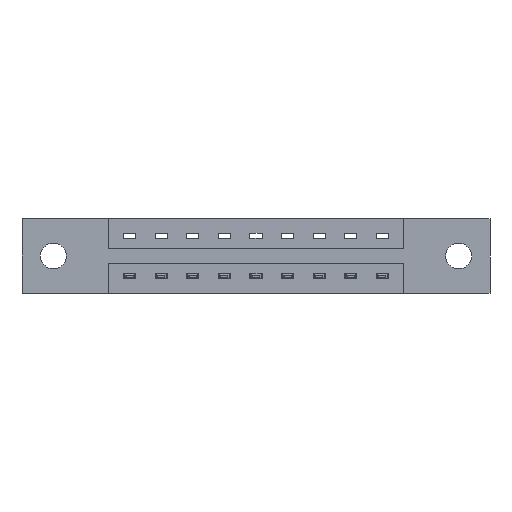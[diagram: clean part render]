
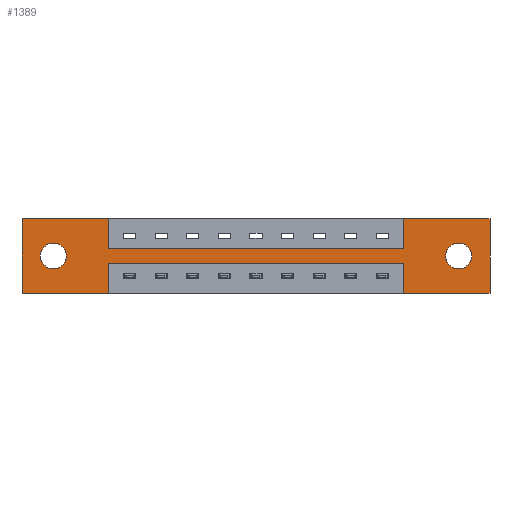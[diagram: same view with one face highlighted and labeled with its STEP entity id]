
A CAD part, front view. The second image highlights one B-rep face of the part: STEP entity #1389.
In plain terms, the highlighted planar face has unit normal (0, -1, 0).
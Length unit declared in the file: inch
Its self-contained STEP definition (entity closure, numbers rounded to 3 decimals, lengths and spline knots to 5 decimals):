
#8 = VECTOR ( 'NONE', #2600, 39.37008 ) ;
#12 = EDGE_CURVE ( 'NONE', #10184, #2739, #1317, .T. ) ;
#14 = EDGE_LOOP ( 'NONE', ( #3819, #10379 ) ) ;
#52 = ORIENTED_EDGE ( 'NONE', *, *, #6218, .T. ) ;
#67 = EDGE_LOOP ( 'NONE', ( #52, #2562 ) ) ;
#458 = VERTEX_POINT ( 'NONE', #7174 ) ;
#569 = EDGE_CURVE ( 'NONE', #7236, #9083, #9987, .T. ) ;
#582 = CARTESIAN_POINT ( 'NONE',  ( 0., 0., 0. ) ) ;
#648 = ORIENTED_EDGE ( 'NONE', *, *, #5419, .F. ) ;
#692 = VECTOR ( 'NONE', #4787, 39.37008 ) ;
#770 = EDGE_CURVE ( 'NONE', #9083, #9207, #10099, .T. ) ;
#872 = VECTOR ( 'NONE', #1946, 39.37008 ) ;
#923 = AXIS2_PLACEMENT_3D ( 'NONE', #2816, #2030, #1575 ) ;
#1024 = CARTESIAN_POINT ( 'NONE',  ( 1.885, 0., 0. ) ) ;
#1047 = CARTESIAN_POINT ( 'NONE',  ( 1.885, 0., -0.15 ) ) ;
#1225 = ORIENTED_EDGE ( 'NONE', *, *, #3499, .F. ) ;
#1302 = CARTESIAN_POINT ( 'NONE',  ( 2.31, 0., 0. ) ) ;
#1317 = LINE ( 'NONE', #1812, #9880 ) ;
#1385 = ORIENTED_EDGE ( 'NONE', *, *, #7901, .F. ) ;
#1389 = ADVANCED_FACE ( 'NONE', ( #9699, #5748, #8130 ), #2143, .T. ) ;
#1575 = DIRECTION ( 'NONE',  ( 0., 0., -1. ) ) ;
#1652 = DIRECTION ( 'NONE',  ( 0., 0., -1. ) ) ;
#1812 = CARTESIAN_POINT ( 'NONE',  ( 1.885, 0., -0.37 ) ) ;
#1946 = DIRECTION ( 'NONE',  ( -1., 0., 0. ) ) ;
#1984 = ORIENTED_EDGE ( 'NONE', *, *, #569, .F. ) ;
#2030 = DIRECTION ( 'NONE',  ( 0., -1., 0. ) ) ;
#2089 = VECTOR ( 'NONE', #8430, 39.37008 ) ;
#2143 = PLANE ( 'NONE',  #923 ) ;
#2194 = VECTOR ( 'NONE', #6625, 39.37008 ) ;
#2396 = CARTESIAN_POINT ( 'NONE',  ( 2.155, 0., -0.185 ) ) ;
#2562 = ORIENTED_EDGE ( 'NONE', *, *, #2701, .T. ) ;
#2600 = DIRECTION ( 'NONE',  ( 0., 0., 1. ) ) ;
#2699 = VERTEX_POINT ( 'NONE', #6415 ) ;
#2701 = EDGE_CURVE ( 'NONE', #4265, #8210, #3915, .T. ) ;
#2739 = VERTEX_POINT ( 'NONE', #5253 ) ;
#2797 = LINE ( 'NONE', #10108, #8 ) ;
#2814 = DIRECTION ( 'NONE',  ( 0., 0., 1. ) ) ;
#2816 = CARTESIAN_POINT ( 'NONE',  ( 0., 0., -0.37 ) ) ;
#2850 = ORIENTED_EDGE ( 'NONE', *, *, #7556, .F. ) ;
#3068 = CARTESIAN_POINT ( 'NONE',  ( 2.155, 0., -0.121 ) ) ;
#3204 = EDGE_CURVE ( 'NONE', #6936, #6884, #4412, .T. ) ;
#3317 = DIRECTION ( 'NONE',  ( 1., 0., 0. ) ) ;
#3389 = DIRECTION ( 'NONE',  ( 1., 0., 0. ) ) ;
#3407 = ORIENTED_EDGE ( 'NONE', *, *, #7855, .F. ) ;
#3423 = EDGE_CURVE ( 'NONE', #2699, #4087, #2797, .T. ) ;
#3446 = DIRECTION ( 'NONE',  ( 0., 0., -1. ) ) ;
#3473 = DIRECTION ( 'NONE',  ( 0., 1., 0. ) ) ;
#3483 = DIRECTION ( 'NONE',  ( 0., 1., 0. ) ) ;
#3499 = EDGE_CURVE ( 'NONE', #7143, #10184, #8337, .T. ) ;
#3549 = DIRECTION ( 'NONE',  ( 0., 0., 1. ) ) ;
#3565 = CIRCLE ( 'NONE', #8037, 0.064 ) ;
#3625 = DIRECTION ( 'NONE',  ( 0., 0., -1. ) ) ;
#3819 = ORIENTED_EDGE ( 'NONE', *, *, #7122, .T. ) ;
#3915 = CIRCLE ( 'NONE', #8149, 0.064 ) ;
#3932 = EDGE_CURVE ( 'NONE', #4850, #9013, #4812, .T. ) ;
#4087 = VERTEX_POINT ( 'NONE', #9113 ) ;
#4117 = CARTESIAN_POINT ( 'NONE',  ( 0.155, 0., -0.121 ) ) ;
#4147 = AXIS2_PLACEMENT_3D ( 'NONE', #2396, #3473, #3446 ) ;
#4148 = CARTESIAN_POINT ( 'NONE',  ( 1.885, 0., -0.37 ) ) ;
#4151 = CARTESIAN_POINT ( 'NONE',  ( 0.155, 0., -0.249 ) ) ;
#4265 = VERTEX_POINT ( 'NONE', #4151 ) ;
#4383 = EDGE_CURVE ( 'NONE', #9013, #7143, #9272, .T. ) ;
#4412 = LINE ( 'NONE', #7427, #2089 ) ;
#4546 = VECTOR ( 'NONE', #6333, 39.37008 ) ;
#4554 = EDGE_CURVE ( 'NONE', #458, #9960, #8317, .T. ) ;
#4787 = DIRECTION ( 'NONE',  ( 1., 0., 0. ) ) ;
#4812 = LINE ( 'NONE', #8941, #5062 ) ;
#4850 = VERTEX_POINT ( 'NONE', #8526 ) ;
#5061 = VECTOR ( 'NONE', #9419, 39.37008 ) ;
#5062 = VECTOR ( 'NONE', #3317, 39.37008 ) ;
#5115 = ORIENTED_EDGE ( 'NONE', *, *, #3204, .F. ) ;
#5125 = ORIENTED_EDGE ( 'NONE', *, *, #3423, .F. ) ;
#5248 = ORIENTED_EDGE ( 'NONE', *, *, #3932, .F. ) ;
#5253 = CARTESIAN_POINT ( 'NONE',  ( 1.885, 0., -0.22 ) ) ;
#5321 = CARTESIAN_POINT ( 'NONE',  ( 0., 0., -0.37 ) ) ;
#5419 = EDGE_CURVE ( 'NONE', #6884, #2699, #9003, .T. ) ;
#5631 = ORIENTED_EDGE ( 'NONE', *, *, #12, .F. ) ;
#5643 = DIRECTION ( 'NONE',  ( 0., 0., 1. ) ) ;
#5748 = FACE_BOUND ( 'NONE', #67, .T. ) ;
#5768 = EDGE_LOOP ( 'NONE', ( #5115, #3407, #5631, #1225, #8258, #5248, #1385, #6011, #1984, #2850, #5125, #648 ) ) ;
#5794 = CARTESIAN_POINT ( 'NONE',  ( 0.425, 0., -0.15 ) ) ;
#5831 = CARTESIAN_POINT ( 'NONE',  ( 0.155, 0., -0.185 ) ) ;
#6011 = ORIENTED_EDGE ( 'NONE', *, *, #770, .F. ) ;
#6160 = CARTESIAN_POINT ( 'NONE',  ( 0., 0., -0.37 ) ) ;
#6218 = EDGE_CURVE ( 'NONE', #8210, #4265, #3565, .T. ) ;
#6225 = CARTESIAN_POINT ( 'NONE',  ( 0.425, 0., -0.22 ) ) ;
#6227 = VECTOR ( 'NONE', #3389, 39.37008 ) ;
#6239 = CIRCLE ( 'NONE', #4147, 0.064 ) ;
#6274 = DIRECTION ( 'NONE',  ( 0., 1., 0. ) ) ;
#6281 = CARTESIAN_POINT ( 'NONE',  ( 0.155, 0., -0.185 ) ) ;
#6333 = DIRECTION ( 'NONE',  ( -1., 0., 0. ) ) ;
#6415 = CARTESIAN_POINT ( 'NONE',  ( 0., 0., -0.37 ) ) ;
#6625 = DIRECTION ( 'NONE',  ( -1., 0., 0. ) ) ;
#6832 = CARTESIAN_POINT ( 'NONE',  ( 2.31, 0., 0. ) ) ;
#6880 = CARTESIAN_POINT ( 'NONE',  ( 0.425, 0., -0.22 ) ) ;
#6884 = VERTEX_POINT ( 'NONE', #10277 ) ;
#6936 = VERTEX_POINT ( 'NONE', #6880 ) ;
#6989 = CARTESIAN_POINT ( 'NONE',  ( 0.425, 0., 0. ) ) ;
#7091 = DIRECTION ( 'NONE',  ( 0., 1., 0. ) ) ;
#7122 = EDGE_CURVE ( 'NONE', #9960, #458, #6239, .T. ) ;
#7143 = VERTEX_POINT ( 'NONE', #7394 ) ;
#7174 = CARTESIAN_POINT ( 'NONE',  ( 2.155, 0., -0.249 ) ) ;
#7234 = VECTOR ( 'NONE', #7875, 39.37008 ) ;
#7236 = VERTEX_POINT ( 'NONE', #10088 ) ;
#7394 = CARTESIAN_POINT ( 'NONE',  ( 2.31, 0., -0.37 ) ) ;
#7427 = CARTESIAN_POINT ( 'NONE',  ( 0.425, 0., -0.37 ) ) ;
#7556 = EDGE_CURVE ( 'NONE', #4087, #7236, #8336, .T. ) ;
#7744 = CARTESIAN_POINT ( 'NONE',  ( 0.425, 0., -0.15 ) ) ;
#7855 = EDGE_CURVE ( 'NONE', #2739, #6936, #9770, .T. ) ;
#7875 = DIRECTION ( 'NONE',  ( 0., 0., -1. ) ) ;
#7901 = EDGE_CURVE ( 'NONE', #9207, #4850, #9541, .T. ) ;
#8037 = AXIS2_PLACEMENT_3D ( 'NONE', #6281, #6274, #5643 ) ;
#8130 = FACE_OUTER_BOUND ( 'NONE', #5768, .T. ) ;
#8149 = AXIS2_PLACEMENT_3D ( 'NONE', #5831, #3483, #3549 ) ;
#8210 = VERTEX_POINT ( 'NONE', #4117 ) ;
#8258 = ORIENTED_EDGE ( 'NONE', *, *, #4383, .F. ) ;
#8317 = CIRCLE ( 'NONE', #10616, 0.064 ) ;
#8336 = LINE ( 'NONE', #582, #6227 ) ;
#8337 = LINE ( 'NONE', #5321, #4546 ) ;
#8430 = DIRECTION ( 'NONE',  ( 0., 0., -1. ) ) ;
#8441 = VECTOR ( 'NONE', #1652, 39.37008 ) ;
#8526 = CARTESIAN_POINT ( 'NONE',  ( 1.885, 0., 0. ) ) ;
#8582 = CARTESIAN_POINT ( 'NONE',  ( 2.155, 0., -0.185 ) ) ;
#8941 = CARTESIAN_POINT ( 'NONE',  ( 0., 0., 0. ) ) ;
#9003 = LINE ( 'NONE', #6160, #2194 ) ;
#9013 = VERTEX_POINT ( 'NONE', #6832 ) ;
#9083 = VERTEX_POINT ( 'NONE', #7744 ) ;
#9113 = CARTESIAN_POINT ( 'NONE',  ( 0., 0., 0. ) ) ;
#9207 = VERTEX_POINT ( 'NONE', #1047 ) ;
#9272 = LINE ( 'NONE', #1302, #7234 ) ;
#9419 = DIRECTION ( 'NONE',  ( 0., 0., 1. ) ) ;
#9541 = LINE ( 'NONE', #1024, #5061 ) ;
#9699 = FACE_BOUND ( 'NONE', #14, .T. ) ;
#9770 = LINE ( 'NONE', #6225, #872 ) ;
#9880 = VECTOR ( 'NONE', #2814, 39.37008 ) ;
#9960 = VERTEX_POINT ( 'NONE', #3068 ) ;
#9987 = LINE ( 'NONE', #6989, #8441 ) ;
#10088 = CARTESIAN_POINT ( 'NONE',  ( 0.425, 0., 0. ) ) ;
#10099 = LINE ( 'NONE', #5794, #692 ) ;
#10108 = CARTESIAN_POINT ( 'NONE',  ( 0., 0., 0. ) ) ;
#10184 = VERTEX_POINT ( 'NONE', #4148 ) ;
#10277 = CARTESIAN_POINT ( 'NONE',  ( 0.425, 0., -0.37 ) ) ;
#10379 = ORIENTED_EDGE ( 'NONE', *, *, #4554, .T. ) ;
#10616 = AXIS2_PLACEMENT_3D ( 'NONE', #8582, #7091, #3625 ) ;
